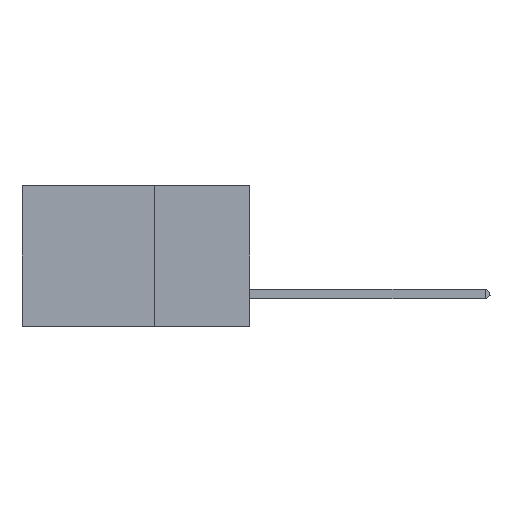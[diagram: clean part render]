
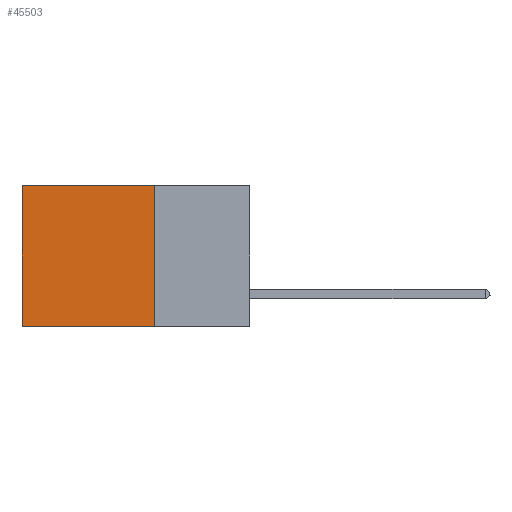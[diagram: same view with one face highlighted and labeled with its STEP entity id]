
A CAD part, left-side view. The second image highlights one B-rep face of the part: STEP entity #45503.
In plain terms, the highlighted planar face has unit normal (-1, 0, 0).
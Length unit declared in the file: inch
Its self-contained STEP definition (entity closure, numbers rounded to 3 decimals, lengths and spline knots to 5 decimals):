
#2000 = DIRECTION ( 'NONE',  ( 0., 0., -1. ) ) ;
#2358 = DIRECTION ( 'NONE',  ( 0., 1., 0. ) ) ;
#5058 = VERTEX_POINT ( 'NONE', #16902 ) ;
#5246 = LINE ( 'NONE', #10269, #48298 ) ;
#6279 = LINE ( 'NONE', #37268, #46916 ) ;
#6857 = CARTESIAN_POINT ( 'NONE',  ( 0.2875, 0.25, -0.37 ) ) ;
#10269 = CARTESIAN_POINT ( 'NONE',  ( 0.2875, 0.6, 0. ) ) ;
#10734 = AXIS2_PLACEMENT_3D ( 'NONE', #28369, #16672, #16511 ) ;
#11263 = VERTEX_POINT ( 'NONE', #6857 ) ;
#13797 = VERTEX_POINT ( 'NONE', #40665 ) ;
#15149 = ORIENTED_EDGE ( 'NONE', *, *, #19669, .T. ) ;
#15234 = ORIENTED_EDGE ( 'NONE', *, *, #42716, .F. ) ;
#16511 = DIRECTION ( 'NONE',  ( 0., 0., -1. ) ) ;
#16672 = DIRECTION ( 'NONE',  ( 1., 0., 0. ) ) ;
#16902 = CARTESIAN_POINT ( 'NONE',  ( 0.2875, 0.6, -0.37 ) ) ;
#19669 = EDGE_CURVE ( 'NONE', #13797, #46233, #34389, .T. ) ;
#21792 = VECTOR ( 'NONE', #2358, 39.37008 ) ;
#23286 = FACE_OUTER_BOUND ( 'NONE', #39413, .T. ) ;
#25262 = EDGE_CURVE ( 'NONE', #46233, #5058, #5246, .T. ) ;
#28369 = CARTESIAN_POINT ( 'NONE',  ( 0.2875, 0.25, 0. ) ) ;
#29835 = CARTESIAN_POINT ( 'NONE',  ( 0.2875, 0.25, 0. ) ) ;
#34389 = LINE ( 'NONE', #29835, #36827 ) ;
#34711 = CARTESIAN_POINT ( 'NONE',  ( 0.2875, 0.6, 0. ) ) ;
#34941 = LINE ( 'NONE', #36442, #21792 ) ;
#35019 = DIRECTION ( 'NONE',  ( 0., 1., 0. ) ) ;
#35574 = ORIENTED_EDGE ( 'NONE', *, *, #25262, .T. ) ;
#36442 = CARTESIAN_POINT ( 'NONE',  ( 0.2875, 0.25, -0.37 ) ) ;
#36827 = VECTOR ( 'NONE', #35019, 39.37008 ) ;
#37268 = CARTESIAN_POINT ( 'NONE',  ( 0.2875, 0.25, 0. ) ) ;
#39413 = EDGE_LOOP ( 'NONE', ( #35574, #15234, #46715, #15149 ) ) ;
#40665 = CARTESIAN_POINT ( 'NONE',  ( 0.2875, 0.25, 0. ) ) ;
#42311 = EDGE_CURVE ( 'NONE', #13797, #11263, #6279, .T. ) ;
#42716 = EDGE_CURVE ( 'NONE', #11263, #5058, #34941, .T. ) ;
#43625 = PLANE ( 'NONE',  #10734 ) ;
#45503 = ADVANCED_FACE ( 'NONE', ( #23286 ), #43625, .F. ) ;
#46233 = VERTEX_POINT ( 'NONE', #34711 ) ;
#46715 = ORIENTED_EDGE ( 'NONE', *, *, #42311, .F. ) ;
#46916 = VECTOR ( 'NONE', #48931, 39.37008 ) ;
#48298 = VECTOR ( 'NONE', #2000, 39.37008 ) ;
#48931 = DIRECTION ( 'NONE',  ( 0., 0., -1. ) ) ;
